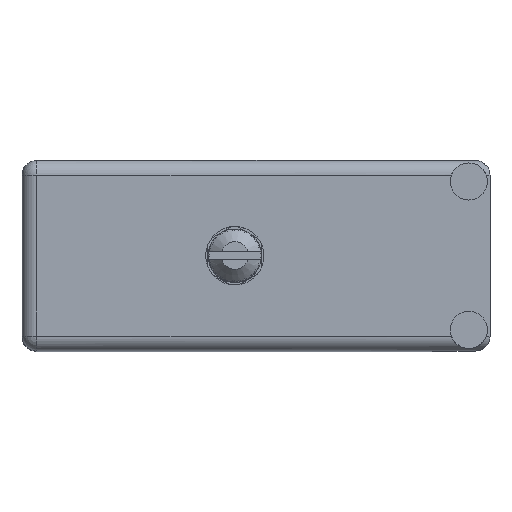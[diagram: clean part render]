
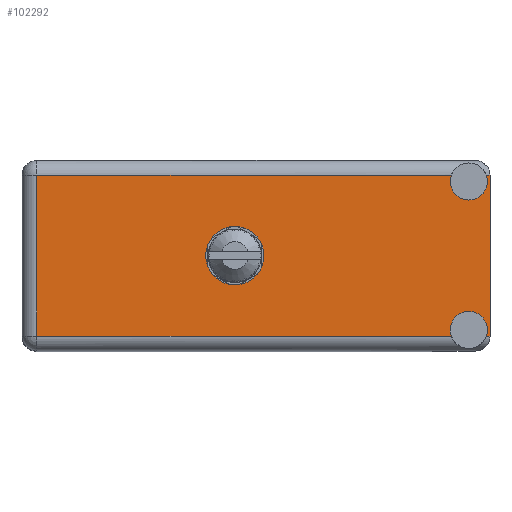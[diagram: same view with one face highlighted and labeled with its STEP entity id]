
A CAD part, top view. The second image highlights one B-rep face of the part: STEP entity #102292.
In plain terms, the highlighted face is planar.
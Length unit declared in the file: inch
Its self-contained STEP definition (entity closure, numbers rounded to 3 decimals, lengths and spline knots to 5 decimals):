
#119 = VERTEX_POINT ( 'NONE', #79260 ) ;
#209 = CARTESIAN_POINT ( 'NONE',  ( 0., 1.566, -0.899 ) ) ;
#280 = FACE_BOUND ( 'NONE', #18317, .T. ) ;
#992 = EDGE_CURVE ( 'NONE', #84880, #68965, #29141, .T. ) ;
#2688 = LINE ( 'NONE', #3449, #104644 ) ;
#2710 = VERTEX_POINT ( 'NONE', #59371 ) ;
#3449 = CARTESIAN_POINT ( 'NONE',  ( 0., 1.566, -0.829 ) ) ;
#3590 = CARTESIAN_POINT ( 'NONE',  ( 0.07, 1.566, -0.829 ) ) ;
#4953 = ORIENTED_EDGE ( 'NONE', *, *, #47682, .F. ) ;
#5404 = AXIS2_PLACEMENT_3D ( 'NONE', #41803, #92116, #7766 ) ;
#5841 = LINE ( 'NONE', #98533, #109212 ) ;
#6474 = LINE ( 'NONE', #28156, #62065 ) ;
#7766 = DIRECTION ( 'NONE',  ( 0., 0., 1. ) ) ;
#8755 = DIRECTION ( 'NONE',  ( 0., 1., 0. ) ) ;
#9429 = EDGE_CURVE ( 'NONE', #23418, #39515, #83706, .T. ) ;
#10009 = DIRECTION ( 'NONE',  ( 0., 0., 1. ) ) ;
#11793 = EDGE_CURVE ( 'NONE', #29478, #23418, #2688, .T. ) ;
#12972 = CIRCLE ( 'NONE', #51953, 0.0875 ) ;
#13130 = LINE ( 'NONE', #26641, #22494 ) ;
#13295 = DIRECTION ( 'NONE',  ( 0., 1., 0. ) ) ;
#14208 = EDGE_CURVE ( 'NONE', #119, #64785, #12972, .T. ) ;
#15830 = CIRCLE ( 'NONE', #22567, 0.0875 ) ;
#17458 = VERTEX_POINT ( 'NONE', #100439 ) ;
#18317 = EDGE_LOOP ( 'NONE', ( #23932, #30617 ) ) ;
#18484 = AXIS2_PLACEMENT_3D ( 'NONE', #30661, #13295, #39196 ) ;
#18553 = LINE ( 'NONE', #69463, #89997 ) ;
#20416 = ORIENTED_EDGE ( 'NONE', *, *, #9429, .T. ) ;
#20598 = CARTESIAN_POINT ( 'NONE',  ( 2.02562, 1.566, -0.829 ) ) ;
#20762 = ORIENTED_EDGE ( 'NONE', *, *, #11793, .T. ) ;
#22494 = VECTOR ( 'NONE', #10009, 39.37008 ) ;
#22567 = AXIS2_PLACEMENT_3D ( 'NONE', #38365, #63851, #71599 ) ;
#23418 = VERTEX_POINT ( 'NONE', #3590 ) ;
#23932 = ORIENTED_EDGE ( 'NONE', *, *, #56223, .F. ) ;
#24610 = EDGE_CURVE ( 'NONE', #17458, #64785, #18553, .T. ) ;
#25341 = EDGE_CURVE ( 'NONE', #17458, #47218, #13130, .T. ) ;
#26641 = CARTESIAN_POINT ( 'NONE',  ( 2.208, 1.566, 0. ) ) ;
#28156 = CARTESIAN_POINT ( 'NONE',  ( 2.208, 1.566, -0.07 ) ) ;
#29141 = CIRCLE ( 'NONE', #83815, 0.1375 ) ;
#29478 = VERTEX_POINT ( 'NONE', #20598 ) ;
#29499 = VECTOR ( 'NONE', #76542, 39.37008 ) ;
#30617 = ORIENTED_EDGE ( 'NONE', *, *, #992, .F. ) ;
#30661 = CARTESIAN_POINT ( 'NONE',  ( 1.004, 1.566, -0.4495 ) ) ;
#32515 = CIRCLE ( 'NONE', #5404, 0.0875 ) ;
#34853 = VERTEX_POINT ( 'NONE', #94554 ) ;
#35123 = DIRECTION ( 'NONE',  ( 0., 1., 0. ) ) ;
#35697 = ORIENTED_EDGE ( 'NONE', *, *, #24610, .T. ) ;
#37618 = VERTEX_POINT ( 'NONE', #57931 ) ;
#38365 = CARTESIAN_POINT ( 'NONE',  ( 2.108, 1.566, -0.0995 ) ) ;
#38529 = CARTESIAN_POINT ( 'NONE',  ( 2.108, 1.566, -0.7995 ) ) ;
#38939 = DIRECTION ( 'NONE',  ( 1., 0., 0. ) ) ;
#39196 = DIRECTION ( 'NONE',  ( 0., 0., 1. ) ) ;
#39515 = VERTEX_POINT ( 'NONE', #66841 ) ;
#41803 = CARTESIAN_POINT ( 'NONE',  ( 2.108, 1.566, -0.0995 ) ) ;
#45213 = DIRECTION ( 'NONE',  ( -1., 0., 0. ) ) ;
#47218 = VERTEX_POINT ( 'NONE', #79154 ) ;
#47590 = ORIENTED_EDGE ( 'NONE', *, *, #77971, .T. ) ;
#47682 = EDGE_CURVE ( 'NONE', #2710, #34853, #15830, .T. ) ;
#49237 = CARTESIAN_POINT ( 'NONE',  ( 2.19038, 1.566, -0.829 ) ) ;
#50523 = PLANE ( 'NONE',  #103630 ) ;
#51953 = AXIS2_PLACEMENT_3D ( 'NONE', #97174, #78994, #62346 ) ;
#54668 = DIRECTION ( 'NONE',  ( -1., 0., 0. ) ) ;
#56223 = EDGE_CURVE ( 'NONE', #68965, #84880, #69092, .T. ) ;
#57931 = CARTESIAN_POINT ( 'NONE',  ( 2.19038, 1.566, -0.07 ) ) ;
#59371 = CARTESIAN_POINT ( 'NONE',  ( 2.108, 1.566, -0.187 ) ) ;
#61422 = DIRECTION ( 'NONE',  ( 1., 0., 0. ) ) ;
#62065 = VECTOR ( 'NONE', #61422, 39.37008 ) ;
#62346 = DIRECTION ( 'NONE',  ( 0., 0., 1. ) ) ;
#62863 = ORIENTED_EDGE ( 'NONE', *, *, #105060, .T. ) ;
#63851 = DIRECTION ( 'NONE',  ( 0., 1., 0. ) ) ;
#64785 = VERTEX_POINT ( 'NONE', #49237 ) ;
#66841 = CARTESIAN_POINT ( 'NONE',  ( 0.07, 1.566, -0.07 ) ) ;
#66939 = CARTESIAN_POINT ( 'NONE',  ( 1.004, 1.566, -0.4495 ) ) ;
#67896 = DIRECTION ( 'NONE',  ( 0., 0., 1. ) ) ;
#68965 = VERTEX_POINT ( 'NONE', #73353 ) ;
#69092 = CIRCLE ( 'NONE', #18484, 0.1375 ) ;
#69463 = CARTESIAN_POINT ( 'NONE',  ( 0., 1.566, -0.829 ) ) ;
#69816 = AXIS2_PLACEMENT_3D ( 'NONE', #38529, #106284, #79187 ) ;
#71599 = DIRECTION ( 'NONE',  ( 0., 0., 1. ) ) ;
#73353 = CARTESIAN_POINT ( 'NONE',  ( 1.004, 1.566, -0.312 ) ) ;
#74801 = CARTESIAN_POINT ( 'NONE',  ( 1.004, 1.566, -0.587 ) ) ;
#75774 = DIRECTION ( 'NONE',  ( 0., 0., 1. ) ) ;
#76542 = DIRECTION ( 'NONE',  ( 0., 0., 1. ) ) ;
#77971 = EDGE_CURVE ( 'NONE', #39515, #34853, #5841, .T. ) ;
#78994 = DIRECTION ( 'NONE',  ( 0., 1., 0. ) ) ;
#79154 = CARTESIAN_POINT ( 'NONE',  ( 2.208, 1.566, -0.07 ) ) ;
#79187 = DIRECTION ( 'NONE',  ( 0., 0., 1. ) ) ;
#79260 = CARTESIAN_POINT ( 'NONE',  ( 2.108, 1.566, -0.712 ) ) ;
#83706 = LINE ( 'NONE', #85102, #29499 ) ;
#83815 = AXIS2_PLACEMENT_3D ( 'NONE', #66939, #35123, #75774 ) ;
#84880 = VERTEX_POINT ( 'NONE', #74801 ) ;
#85102 = CARTESIAN_POINT ( 'NONE',  ( 0.07, 1.566, -0.899 ) ) ;
#87809 = ORIENTED_EDGE ( 'NONE', *, *, #91616, .F. ) ;
#89455 = CIRCLE ( 'NONE', #69816, 0.0875 ) ;
#89873 = ORIENTED_EDGE ( 'NONE', *, *, #91529, .F. ) ;
#89997 = VECTOR ( 'NONE', #54668, 39.37008 ) ;
#91529 = EDGE_CURVE ( 'NONE', #29478, #119, #89455, .T. ) ;
#91616 = EDGE_CURVE ( 'NONE', #37618, #2710, #32515, .T. ) ;
#92116 = DIRECTION ( 'NONE',  ( 0., 1., 0. ) ) ;
#94554 = CARTESIAN_POINT ( 'NONE',  ( 2.02562, 1.566, -0.07 ) ) ;
#96950 = FACE_OUTER_BOUND ( 'NONE', #103826, .T. ) ;
#97174 = CARTESIAN_POINT ( 'NONE',  ( 2.108, 1.566, -0.7995 ) ) ;
#98533 = CARTESIAN_POINT ( 'NONE',  ( 2.208, 1.566, -0.07 ) ) ;
#98748 = ORIENTED_EDGE ( 'NONE', *, *, #14208, .F. ) ;
#100439 = CARTESIAN_POINT ( 'NONE',  ( 2.208, 1.566, -0.829 ) ) ;
#102292 = ADVANCED_FACE ( 'NONE', ( #280, #96950 ), #50523, .T. ) ;
#103630 = AXIS2_PLACEMENT_3D ( 'NONE', #209, #8755, #67896 ) ;
#103826 = EDGE_LOOP ( 'NONE', ( #47590, #4953, #87809, #62863, #105297, #35697, #98748, #89873, #20762, #20416 ) ) ;
#104644 = VECTOR ( 'NONE', #45213, 39.37008 ) ;
#105060 = EDGE_CURVE ( 'NONE', #37618, #47218, #6474, .T. ) ;
#105297 = ORIENTED_EDGE ( 'NONE', *, *, #25341, .F. ) ;
#106284 = DIRECTION ( 'NONE',  ( 0., 1., 0. ) ) ;
#109212 = VECTOR ( 'NONE', #38939, 39.37008 ) ;
